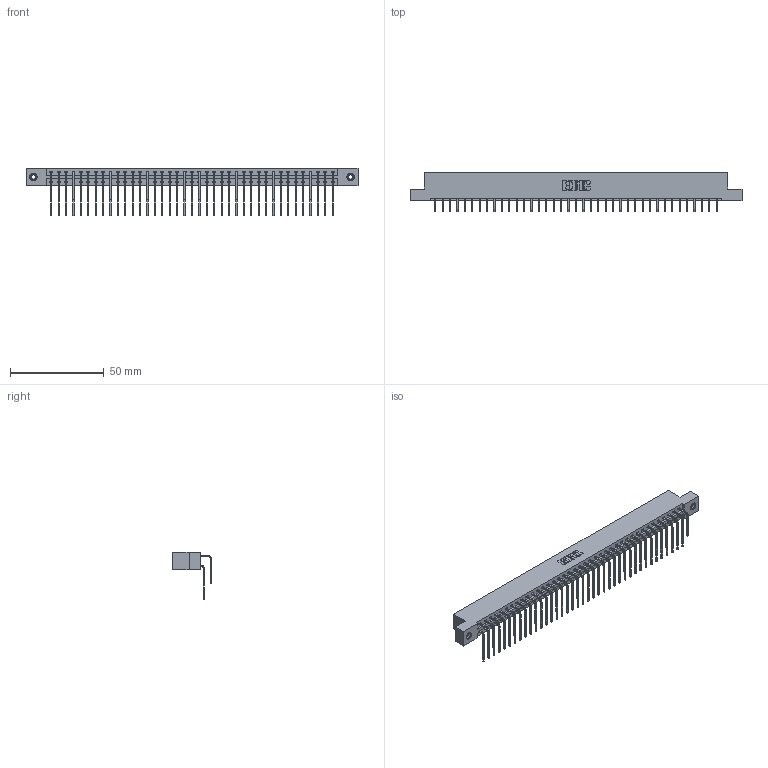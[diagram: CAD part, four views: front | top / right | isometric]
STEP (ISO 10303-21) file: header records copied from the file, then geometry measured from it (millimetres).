
FILE_DESCRIPTION (( 'STEP AP203' ), '1' );
FILE_NAME ('387-078-559-208.STEP', '2019-10-22T07:10:44', ( '' ), ( '' ), 'SwSTEP 2.0', 'SolidWorks 2016', '' );
FILE_SCHEMA (( 'CONFIG_CONTROL_DESIGN' ));
Length unit declared in the file: inch
Products named in the file (5): 337 Part_Flush Mounting Lugs - 0.156 Dia-TI; 345-250-001_345-250-003-102; 345-292-001_559 Tail - 2; 345-292-001_558 559 Tail - 1; 387-078-559-208
Assembly tree (81 placements, depth 2):
  387-078-559-208
    337 Part_Flush Mounting Lugs - 0.156 Dia-TI
    345-292-001_558 559 Tail - 1  x39
    345-292-001_559 Tail - 2  x39
    345-250-001_345-250-003-102  x2
Bounding box: 177.55 x 20.9 x 25.53 mm (x, y, z)
Volume: 19114.7 mm3; surface area: 23863.4 mm2
Topology: 81 solids, 81 shells, 4542 faces, 13473 edges, 8870 vertices
Faces by surface type: plane 3222, cylinder 1304, cone 12, torus 4
Entity records: 33596 total; most frequent: CARTESIAN_POINT 5688, ORIENTED_EDGE 5566, DIRECTION 4857, EDGE_CURVE 2783, LINE 2595, VECTOR 2595, VERTEX_POINT 1848, AXIS2_PLACEMENT_3D 1131
